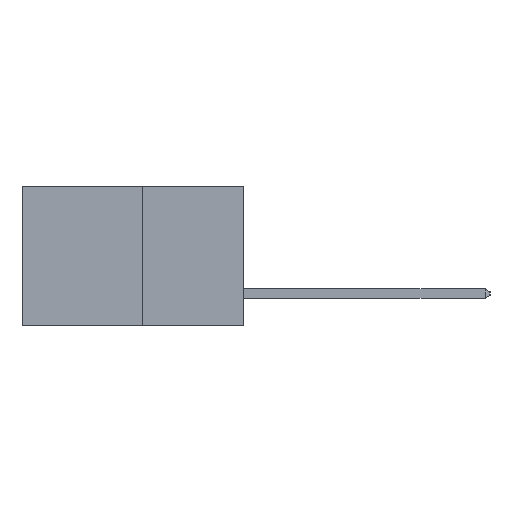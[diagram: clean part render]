
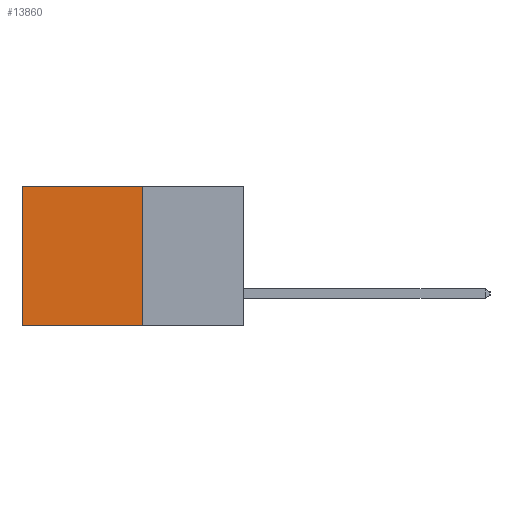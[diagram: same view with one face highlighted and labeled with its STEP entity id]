
A CAD part, left-side view. The second image highlights one B-rep face of the part: STEP entity #13860.
In plain terms, the highlighted planar face has unit normal (-1, 0, 0).
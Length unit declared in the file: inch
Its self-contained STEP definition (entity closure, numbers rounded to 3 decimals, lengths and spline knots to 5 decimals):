
#450 = FACE_OUTER_BOUND ( 'NONE', #4441, .T. ) ;
#503 = AXIS2_PLACEMENT_3D ( 'NONE', #7569, #16165, #8812 ) ;
#791 = LINE ( 'NONE', #8193, #7749 ) ;
#1137 = VERTEX_POINT ( 'NONE', #4938 ) ;
#1509 = CARTESIAN_POINT ( 'NONE',  ( 0.277, 0.59, -0.37 ) ) ;
#1624 = LINE ( 'NONE', #12150, #14358 ) ;
#1778 = CARTESIAN_POINT ( 'NONE',  ( 0.277, 0.59, 0. ) ) ;
#3004 = DIRECTION ( 'NONE',  ( 0., 0., -1. ) ) ;
#3061 = EDGE_CURVE ( 'NONE', #1137, #13616, #791, .T. ) ;
#3363 = VERTEX_POINT ( 'NONE', #1509 ) ;
#3873 = ORIENTED_EDGE ( 'NONE', *, *, #3061, .F. ) ;
#3972 = LINE ( 'NONE', #5235, #13619 ) ;
#4317 = ORIENTED_EDGE ( 'NONE', *, *, #6932, .T. ) ;
#4441 = EDGE_LOOP ( 'NONE', ( #9843, #13535, #3873, #4317 ) ) ;
#4938 = CARTESIAN_POINT ( 'NONE',  ( 0.277, 0.27, 0. ) ) ;
#5001 = DIRECTION ( 'NONE',  ( 0., 1., 0. ) ) ;
#5235 = CARTESIAN_POINT ( 'NONE',  ( 0.277, 0.27, 0. ) ) ;
#5756 = DIRECTION ( 'NONE',  ( 0., 1., 0. ) ) ;
#6932 = EDGE_CURVE ( 'NONE', #1137, #7226, #3972, .T. ) ;
#7226 = VERTEX_POINT ( 'NONE', #1778 ) ;
#7569 = CARTESIAN_POINT ( 'NONE',  ( 0.277, 0.27, -0.37 ) ) ;
#7749 = VECTOR ( 'NONE', #3004, 39.37008 ) ;
#8193 = CARTESIAN_POINT ( 'NONE',  ( 0.277, 0.27, -0.37 ) ) ;
#8387 = CARTESIAN_POINT ( 'NONE',  ( 0.277, 0.27, -0.37 ) ) ;
#8812 = DIRECTION ( 'NONE',  ( 0., 0., -1. ) ) ;
#9061 = LINE ( 'NONE', #11985, #11995 ) ;
#9843 = ORIENTED_EDGE ( 'NONE', *, *, #15021, .T. ) ;
#10747 = EDGE_CURVE ( 'NONE', #13616, #3363, #9061, .T. ) ;
#11985 = CARTESIAN_POINT ( 'NONE',  ( 0.277, 0.27, -0.37 ) ) ;
#11995 = VECTOR ( 'NONE', #5756, 39.37008 ) ;
#12150 = CARTESIAN_POINT ( 'NONE',  ( 0.277, 0.59, -0.37 ) ) ;
#13535 = ORIENTED_EDGE ( 'NONE', *, *, #10747, .F. ) ;
#13616 = VERTEX_POINT ( 'NONE', #8387 ) ;
#13619 = VECTOR ( 'NONE', #5001, 39.37008 ) ;
#13860 = ADVANCED_FACE ( 'NONE', ( #450 ), #14986, .F. ) ;
#14358 = VECTOR ( 'NONE', #14634, 39.37008 ) ;
#14634 = DIRECTION ( 'NONE',  ( 0., 0., -1. ) ) ;
#14986 = PLANE ( 'NONE',  #503 ) ;
#15021 = EDGE_CURVE ( 'NONE', #7226, #3363, #1624, .T. ) ;
#16165 = DIRECTION ( 'NONE',  ( 1., 0., 0. ) ) ;
